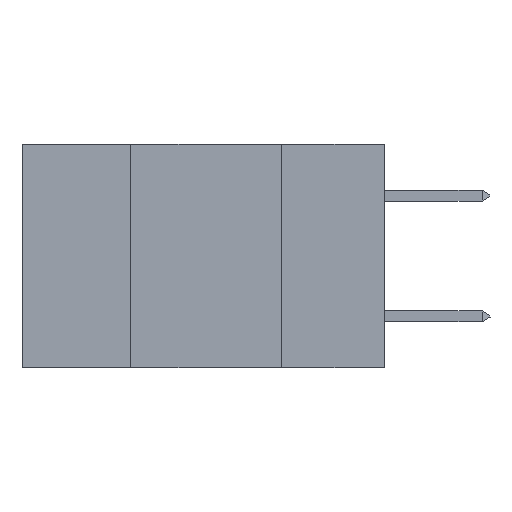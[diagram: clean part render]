
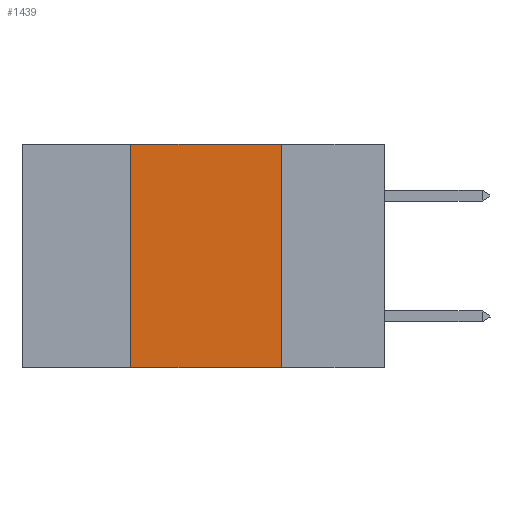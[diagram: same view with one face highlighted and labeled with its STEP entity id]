
A CAD part, left-side view. The second image highlights one B-rep face of the part: STEP entity #1439.
In plain terms, the highlighted planar face has unit normal (-1, 0, 0).
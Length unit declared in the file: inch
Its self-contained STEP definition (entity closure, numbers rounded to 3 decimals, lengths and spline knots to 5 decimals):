
#1340 = CARTESIAN_POINT ( 'NONE',  ( 0., 0.17, -0.37 ) ) ;
#1423 = LINE ( 'NONE', #14136, #6887 ) ;
#1439 = ADVANCED_FACE ( 'NONE', ( #10742 ), #4855, .F. ) ;
#1700 = LINE ( 'NONE', #13637, #7163 ) ;
#1806 = VERTEX_POINT ( 'NONE', #7918 ) ;
#1964 = DIRECTION ( 'NONE',  ( 0., 0., 1. ) ) ;
#2078 = CARTESIAN_POINT ( 'NONE',  ( 0., 0.17, 0. ) ) ;
#2166 = VERTEX_POINT ( 'NONE', #2078 ) ;
#2629 = ORIENTED_EDGE ( 'NONE', *, *, #7285, .T. ) ;
#3336 = VECTOR ( 'NONE', #7530, 39.37008 ) ;
#3466 = CARTESIAN_POINT ( 'NONE',  ( 0., 0.6, 0. ) ) ;
#3810 = ORIENTED_EDGE ( 'NONE', *, *, #12866, .F. ) ;
#3812 = DIRECTION ( 'NONE',  ( 0., 0., -1. ) ) ;
#4214 = ORIENTED_EDGE ( 'NONE', *, *, #5156, .F. ) ;
#4381 = VECTOR ( 'NONE', #6293, 39.37008 ) ;
#4792 = ORIENTED_EDGE ( 'NONE', *, *, #9615, .F. ) ;
#4855 = PLANE ( 'NONE',  #6498 ) ;
#5156 = EDGE_CURVE ( 'NONE', #6958, #2166, #9696, .T. ) ;
#5168 = CARTESIAN_POINT ( 'NONE',  ( 0., 0.6, -0.37 ) ) ;
#6293 = DIRECTION ( 'NONE',  ( 0., -1., 0. ) ) ;
#6498 = AXIS2_PLACEMENT_3D ( 'NONE', #3466, #13837, #13460 ) ;
#6887 = VECTOR ( 'NONE', #1964, 39.37008 ) ;
#6958 = VERTEX_POINT ( 'NONE', #13308 ) ;
#7163 = VECTOR ( 'NONE', #3812, 39.37008 ) ;
#7285 = EDGE_CURVE ( 'NONE', #1806, #10957, #8139, .T. ) ;
#7530 = DIRECTION ( 'NONE',  ( 0., -1., 0. ) ) ;
#7918 = CARTESIAN_POINT ( 'NONE',  ( 0., 0.42, -0.37 ) ) ;
#7946 = CARTESIAN_POINT ( 'NONE',  ( 0., 0.6, 0. ) ) ;
#8139 = LINE ( 'NONE', #5168, #4381 ) ;
#9615 = EDGE_CURVE ( 'NONE', #2166, #10957, #1700, .T. ) ;
#9696 = LINE ( 'NONE', #7946, #3336 ) ;
#10742 = FACE_OUTER_BOUND ( 'NONE', #11886, .T. ) ;
#10957 = VERTEX_POINT ( 'NONE', #1340 ) ;
#11886 = EDGE_LOOP ( 'NONE', ( #4792, #4214, #3810, #2629 ) ) ;
#12866 = EDGE_CURVE ( 'NONE', #1806, #6958, #1423, .T. ) ;
#13308 = CARTESIAN_POINT ( 'NONE',  ( 0., 0.42, 0. ) ) ;
#13460 = DIRECTION ( 'NONE',  ( 0., 0., -1. ) ) ;
#13637 = CARTESIAN_POINT ( 'NONE',  ( 0., 0.17, 0. ) ) ;
#13837 = DIRECTION ( 'NONE',  ( 1., 0., 0. ) ) ;
#14136 = CARTESIAN_POINT ( 'NONE',  ( 0., 0.42, 0. ) ) ;
